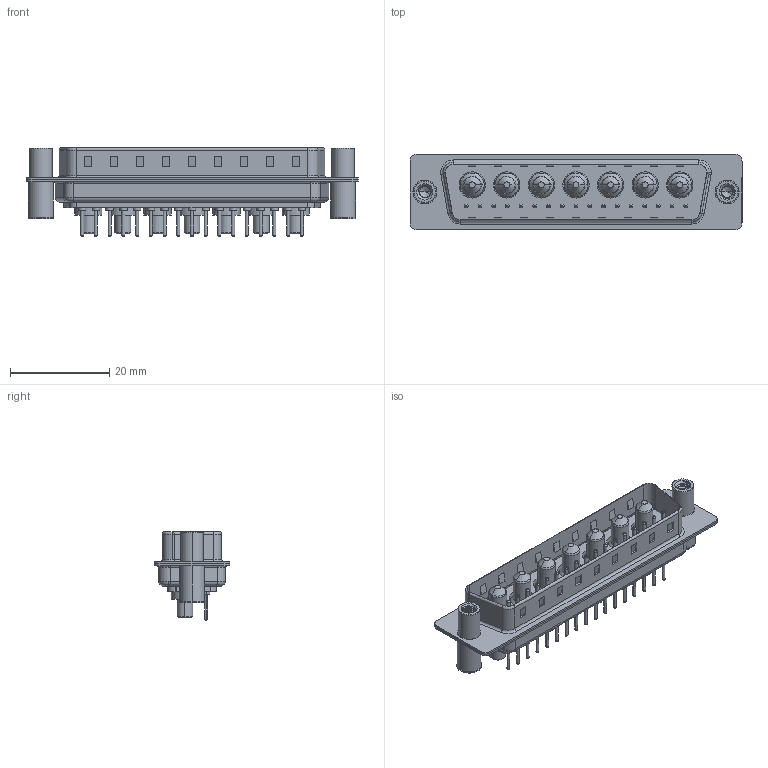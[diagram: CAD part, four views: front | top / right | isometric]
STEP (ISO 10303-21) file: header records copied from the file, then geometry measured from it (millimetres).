
FILE_DESCRIPTION (( 'STEP AP203' ), '1' );
FILE_NAME ('627-24W7624-3NC.STEP', '2019-06-19T00:12:36', ( '' ), ( '' ), 'SwSTEP 2.0', 'SolidWorks 2016', '' );
FILE_SCHEMA (( 'CONFIG_CONTROL_DESIGN' ));
Length unit declared in the file: millimetre
Products named in the file (8): 627Combo Housing_24W7; 627Combo Shell Rear_50 Contacts; 627Combo Shell Front_50 Contacts; 627Combo Threaded Standoff and Board Spacer_C; Power Pin_30A S; 627Combo Threaded Standoff and Board Spacer_4; 627Combo Contact Row 3_24; 627-24W7624-3NC
Assembly tree (29 placements, depth 2):
  627-24W7624-3NC
    627Combo Housing_24W7
    627Combo Shell Rear_50 Contacts
    627Combo Shell Front_50 Contacts
    627Combo Threaded Standoff and Board Spacer_C
    Power Pin_30A S  x7
    627Combo Threaded Standoff and Board Spacer_4
    627Combo Contact Row 3_24  x17
Bounding box: 67 x 15.3 x 17.9 mm (x, y, z)
Volume: 5351.8 mm3; surface area: 11181.1 mm2
Topology: 36 solids, 36 shells, 1416 faces, 3156 edges, 1927 vertices
Faces by surface type: cylinder 574, plane 398, torus 340, cone 78, bspline 26
Entity records: 28129 total; most frequent: CARTESIAN_POINT 8910, DIRECTION 3853, ORIENTED_EDGE 3624, EDGE_CURVE 1812, AXIS2_PLACEMENT_3D 1473, VERTEX_POINT 1151, VECTOR 907, LINE 907
